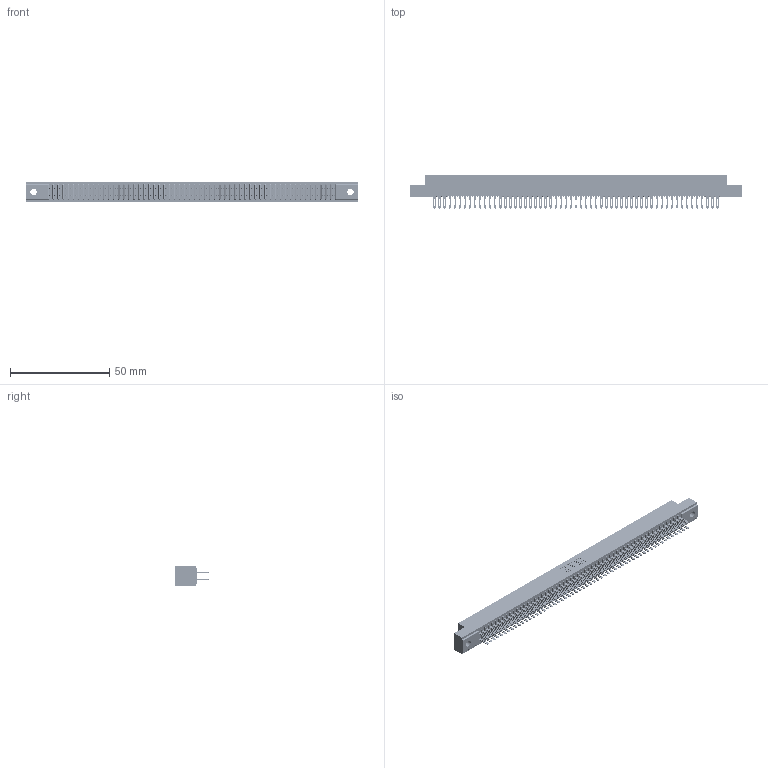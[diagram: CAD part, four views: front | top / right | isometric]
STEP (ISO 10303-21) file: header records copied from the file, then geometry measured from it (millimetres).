
FILE_DESCRIPTION (( 'STEP AP203' ), '1' );
FILE_NAME ('341-114-500-202.STEP', '2018-08-08T13:22:17', ( '' ), ( '' ), 'SwSTEP 2.0', 'SolidWorks 2016', '' );
FILE_SCHEMA (( 'CONFIG_CONTROL_DESIGN' ));
Products named in the file (3): 341-292-001_341-292-100; 341-114-500-202; 341 Part_.128 (3.25) Dia Mounting Holes
Assembly tree (115 placements, depth 2):
  341-114-500-202
    341 Part_.128 (3.25) Dia Mounting Holes
    341-292-001_341-292-100  x114
Bounding box: 167 x 16.69 x 10.16 mm (x, y, z)
Volume: 12452.8 mm3; surface area: 23278.5 mm2
Topology: 115 solids, 115 shells, 7640 faces, 22147 edges, 14342 vertices
Faces by surface type: plane 4400, cylinder 3012, sphere 116, torus 112
Entity records: 66994 total; most frequent: CARTESIAN_POINT 11135, ORIENTED_EDGE 11066, DIRECTION 10799, EDGE_CURVE 5533, VECTOR 4483, LINE 4483, VERTEX_POINT 3494, AXIS2_PLACEMENT_3D 3158
